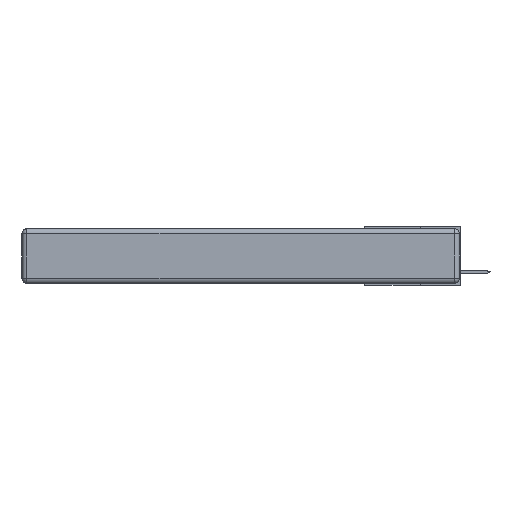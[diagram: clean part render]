
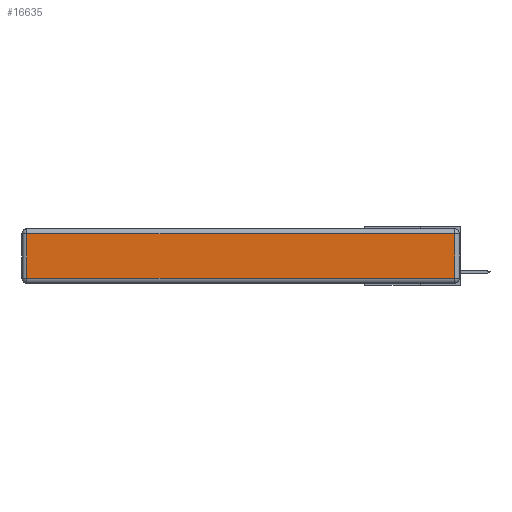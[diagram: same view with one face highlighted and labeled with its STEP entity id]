
A CAD part, left-side view. The second image highlights one B-rep face of the part: STEP entity #16635.
In plain terms, the highlighted planar face has unit normal (-1, 0, 0).
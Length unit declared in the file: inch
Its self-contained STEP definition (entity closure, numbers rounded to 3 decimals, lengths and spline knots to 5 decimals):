
#1236 = DIRECTION ( 'NONE',  ( 0., 0., 1. ) ) ;
#1911 = VECTOR ( 'NONE', #27793, 39.37008 ) ;
#3028 = CARTESIAN_POINT ( 'NONE',  ( 0., 2.75, -0.03 ) ) ;
#3671 = ORIENTED_EDGE ( 'NONE', *, *, #24848, .T. ) ;
#4902 = VECTOR ( 'NONE', #26169, 39.37008 ) ;
#6367 = LINE ( 'NONE', #7329, #1911 ) ;
#7329 = CARTESIAN_POINT ( 'NONE',  ( 0., 0., -0.313 ) ) ;
#7547 = CARTESIAN_POINT ( 'NONE',  ( 0., 0.03, -0.313 ) ) ;
#8069 = FACE_OUTER_BOUND ( 'NONE', #33300, .T. ) ;
#9373 = ORIENTED_EDGE ( 'NONE', *, *, #32910, .T. ) ;
#12405 = PLANE ( 'NONE',  #20864 ) ;
#13364 = VECTOR ( 'NONE', #1236, 39.37008 ) ;
#15116 = CARTESIAN_POINT ( 'NONE',  ( 0., 2.72, -0.313 ) ) ;
#15687 = CARTESIAN_POINT ( 'NONE',  ( 0., 0., -0.343 ) ) ;
#16635 = ADVANCED_FACE ( 'NONE', ( #8069 ), #12405, .T. ) ;
#16793 = CARTESIAN_POINT ( 'NONE',  ( 0., 0.03, -0.343 ) ) ;
#17612 = VERTEX_POINT ( 'NONE', #15116 ) ;
#17760 = VERTEX_POINT ( 'NONE', #20381 ) ;
#19818 = ORIENTED_EDGE ( 'NONE', *, *, #30713, .T. ) ;
#20381 = CARTESIAN_POINT ( 'NONE',  ( 0., 0.03, -0.03 ) ) ;
#20864 = AXIS2_PLACEMENT_3D ( 'NONE', #15687, #21049, #29495 ) ;
#21049 = DIRECTION ( 'NONE',  ( -1., 0., 0. ) ) ;
#22540 = ORIENTED_EDGE ( 'NONE', *, *, #29307, .T. ) ;
#23672 = LINE ( 'NONE', #3028, #28121 ) ;
#24848 = EDGE_CURVE ( 'NONE', #26124, #17760, #27102, .T. ) ;
#26051 = CARTESIAN_POINT ( 'NONE',  ( 0., 2.72, -0.343 ) ) ;
#26097 = DIRECTION ( 'NONE',  ( 0., 1., 0. ) ) ;
#26124 = VERTEX_POINT ( 'NONE', #7547 ) ;
#26169 = DIRECTION ( 'NONE',  ( 0., 0., -1. ) ) ;
#27102 = LINE ( 'NONE', #16793, #13364 ) ;
#27146 = LINE ( 'NONE', #26051, #4902 ) ;
#27793 = DIRECTION ( 'NONE',  ( 0., -1., 0. ) ) ;
#28121 = VECTOR ( 'NONE', #26097, 39.37008 ) ;
#29307 = EDGE_CURVE ( 'NONE', #17612, #26124, #6367, .T. ) ;
#29495 = DIRECTION ( 'NONE',  ( 0., 0., 1. ) ) ;
#30713 = EDGE_CURVE ( 'NONE', #17760, #31666, #23672, .T. ) ;
#31666 = VERTEX_POINT ( 'NONE', #31924 ) ;
#31924 = CARTESIAN_POINT ( 'NONE',  ( 0., 2.72, -0.03 ) ) ;
#32910 = EDGE_CURVE ( 'NONE', #31666, #17612, #27146, .T. ) ;
#33300 = EDGE_LOOP ( 'NONE', ( #22540, #3671, #19818, #9373 ) ) ;
